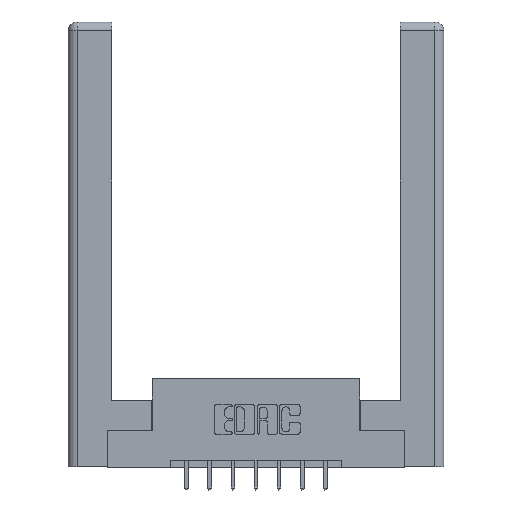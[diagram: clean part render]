
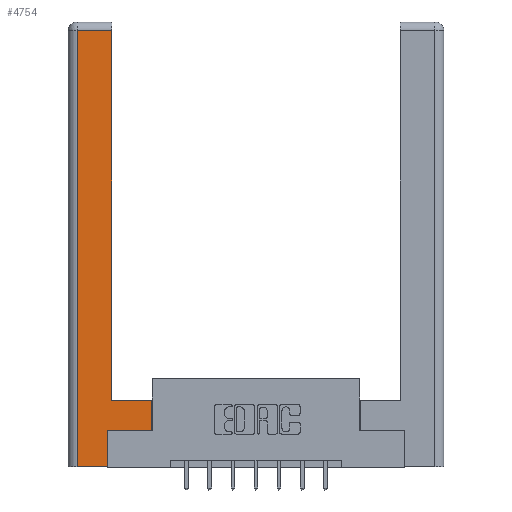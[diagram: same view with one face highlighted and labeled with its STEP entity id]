
A CAD part, top view. The second image highlights one B-rep face of the part: STEP entity #4754.
In plain terms, the highlighted planar face has unit normal (0, 0, 1).
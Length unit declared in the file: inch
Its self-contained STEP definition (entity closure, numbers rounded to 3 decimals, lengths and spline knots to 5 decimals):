
#227 = VECTOR ( 'NONE', #4063, 39.37008 ) ;
#526 = LINE ( 'NONE', #7975, #227 ) ;
#927 = LINE ( 'NONE', #6284, #12201 ) ;
#946 = EDGE_CURVE ( 'NONE', #1785, #12500, #11988, .T. ) ;
#1063 = EDGE_CURVE ( 'NONE', #3794, #6521, #3749, .T. ) ;
#1071 = DIRECTION ( 'NONE',  ( 0., 1., 0. ) ) ;
#1179 = VECTOR ( 'NONE', #2008, 39.37008 ) ;
#1785 = VERTEX_POINT ( 'NONE', #3150 ) ;
#1841 = CARTESIAN_POINT ( 'NONE',  ( 0.565, 0.45, 0. ) ) ;
#2008 = DIRECTION ( 'NONE',  ( 1., 0., 0. ) ) ;
#2472 = CARTESIAN_POINT ( 'NONE',  ( 0.565, 0.45, 0. ) ) ;
#2500 = EDGE_CURVE ( 'NONE', #8312, #7096, #9359, .T. ) ;
#2856 = ORIENTED_EDGE ( 'NONE', *, *, #7577, .T. ) ;
#2929 = LINE ( 'NONE', #6571, #12240 ) ;
#3150 = CARTESIAN_POINT ( 'NONE',  ( 0.295, 0.45, 0. ) ) ;
#3749 = LINE ( 'NONE', #9802, #1179 ) ;
#3794 = VERTEX_POINT ( 'NONE', #10354 ) ;
#3816 = VERTEX_POINT ( 'NONE', #11888 ) ;
#4063 = DIRECTION ( 'NONE',  ( -1., 0., 0. ) ) ;
#4498 = EDGE_CURVE ( 'NONE', #12500, #3816, #5692, .T. ) ;
#4754 = ADVANCED_FACE ( 'NONE', ( #11409 ), #6397, .F. ) ;
#5041 = VERTEX_POINT ( 'NONE', #11524 ) ;
#5374 = CARTESIAN_POINT ( 'NONE',  ( 0., 0., 0. ) ) ;
#5692 = LINE ( 'NONE', #5735, #9833 ) ;
#5735 = CARTESIAN_POINT ( 'NONE',  ( 0.0615, 2.94, 0. ) ) ;
#5838 = VECTOR ( 'NONE', #1071, 39.37008 ) ;
#6284 = CARTESIAN_POINT ( 'NONE',  ( 0.565, 0.245, 0. ) ) ;
#6311 = ORIENTED_EDGE ( 'NONE', *, *, #1063, .T. ) ;
#6369 = DIRECTION ( 'NONE',  ( 0., 1., 0. ) ) ;
#6397 = PLANE ( 'NONE',  #11104 ) ;
#6521 = VERTEX_POINT ( 'NONE', #11954 ) ;
#6571 = CARTESIAN_POINT ( 'NONE',  ( 0.0615, 0., 0. ) ) ;
#6699 = EDGE_CURVE ( 'NONE', #7096, #1785, #526, .T. ) ;
#6742 = VECTOR ( 'NONE', #11245, 39.37008 ) ;
#6839 = ORIENTED_EDGE ( 'NONE', *, *, #4498, .T. ) ;
#7096 = VERTEX_POINT ( 'NONE', #1841 ) ;
#7214 = LINE ( 'NONE', #9893, #5838 ) ;
#7577 = EDGE_CURVE ( 'NONE', #3816, #3794, #2929, .T. ) ;
#7593 = DIRECTION ( 'NONE',  ( 0., -1., 0. ) ) ;
#7975 = CARTESIAN_POINT ( 'NONE',  ( 0.295, 0.45, 0. ) ) ;
#8202 = ORIENTED_EDGE ( 'NONE', *, *, #12508, .T. ) ;
#8312 = VERTEX_POINT ( 'NONE', #10289 ) ;
#8370 = ORIENTED_EDGE ( 'NONE', *, *, #2500, .T. ) ;
#8791 = VECTOR ( 'NONE', #6369, 39.37008 ) ;
#8867 = CARTESIAN_POINT ( 'NONE',  ( 0.295, 2.94, 0. ) ) ;
#9117 = DIRECTION ( 'NONE',  ( 1., 0., 0. ) ) ;
#9264 = ORIENTED_EDGE ( 'NONE', *, *, #9676, .T. ) ;
#9359 = LINE ( 'NONE', #2472, #6742 ) ;
#9465 = ORIENTED_EDGE ( 'NONE', *, *, #6699, .T. ) ;
#9676 = EDGE_CURVE ( 'NONE', #5041, #8312, #927, .T. ) ;
#9802 = CARTESIAN_POINT ( 'NONE',  ( 0.265, 0., 0. ) ) ;
#9833 = VECTOR ( 'NONE', #12589, 39.37008 ) ;
#9893 = CARTESIAN_POINT ( 'NONE',  ( 0.265, 0.245, 0. ) ) ;
#10090 = ORIENTED_EDGE ( 'NONE', *, *, #946, .T. ) ;
#10289 = CARTESIAN_POINT ( 'NONE',  ( 0.565, 0.245, 0. ) ) ;
#10292 = DIRECTION ( 'NONE',  ( 0., 0., -1. ) ) ;
#10354 = CARTESIAN_POINT ( 'NONE',  ( 0.0615, 0., 0. ) ) ;
#11064 = EDGE_LOOP ( 'NONE', ( #10090, #6839, #2856, #6311, #8202, #9264, #8370, #9465 ) ) ;
#11104 = AXIS2_PLACEMENT_3D ( 'NONE', #5374, #10292, #12221 ) ;
#11245 = DIRECTION ( 'NONE',  ( 0., 1., 0. ) ) ;
#11409 = FACE_OUTER_BOUND ( 'NONE', #11064, .T. ) ;
#11524 = CARTESIAN_POINT ( 'NONE',  ( 0.265, 0.245, 0. ) ) ;
#11888 = CARTESIAN_POINT ( 'NONE',  ( 0.0615, 2.94, 0. ) ) ;
#11954 = CARTESIAN_POINT ( 'NONE',  ( 0.265, 0., 0. ) ) ;
#11988 = LINE ( 'NONE', #12186, #8791 ) ;
#12186 = CARTESIAN_POINT ( 'NONE',  ( 0.295, 3., 0. ) ) ;
#12201 = VECTOR ( 'NONE', #9117, 39.37008 ) ;
#12221 = DIRECTION ( 'NONE',  ( -1., 0., 0. ) ) ;
#12240 = VECTOR ( 'NONE', #7593, 39.37008 ) ;
#12500 = VERTEX_POINT ( 'NONE', #8867 ) ;
#12508 = EDGE_CURVE ( 'NONE', #6521, #5041, #7214, .T. ) ;
#12589 = DIRECTION ( 'NONE',  ( -1., 0., 0. ) ) ;
